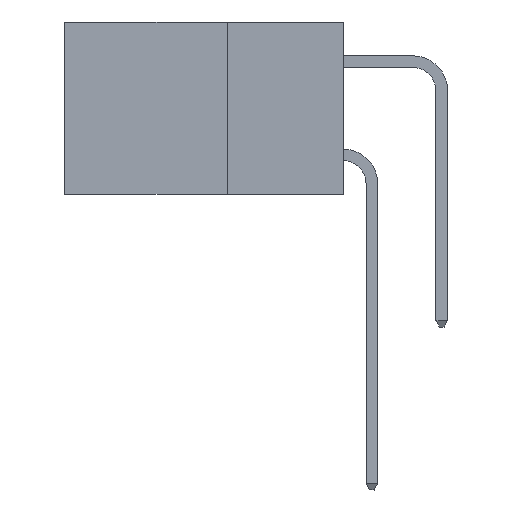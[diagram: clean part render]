
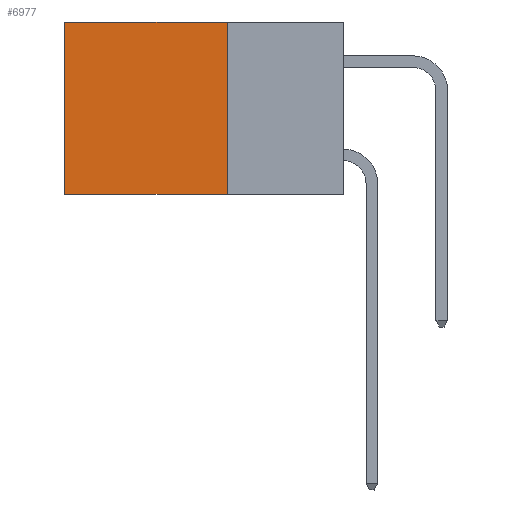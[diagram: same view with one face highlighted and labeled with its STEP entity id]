
A CAD part, left-side view. The second image highlights one B-rep face of the part: STEP entity #6977.
In plain terms, the highlighted planar face has unit normal (-1, 0, 0).
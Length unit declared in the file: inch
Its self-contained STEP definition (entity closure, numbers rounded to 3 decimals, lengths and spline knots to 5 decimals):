
#187 = CARTESIAN_POINT ( 'NONE',  ( 0.2615, 0.25, -0.37 ) ) ;
#285 = LINE ( 'NONE', #5379, #15265 ) ;
#374 = DIRECTION ( 'NONE',  ( 1., 0., 0. ) ) ;
#915 = CARTESIAN_POINT ( 'NONE',  ( 0.2615, 0.25, 0. ) ) ;
#1106 = ORIENTED_EDGE ( 'NONE', *, *, #14473, .T. ) ;
#1327 = DIRECTION ( 'NONE',  ( 0., 0., -1. ) ) ;
#1402 = ORIENTED_EDGE ( 'NONE', *, *, #2349, .F. ) ;
#2270 = VECTOR ( 'NONE', #15679, 39.37008 ) ;
#2349 = EDGE_CURVE ( 'NONE', #12914, #11816, #2787, .T. ) ;
#2787 = LINE ( 'NONE', #6552, #2270 ) ;
#3125 = DIRECTION ( 'NONE',  ( 0., 0., -1. ) ) ;
#4162 = VECTOR ( 'NONE', #15305, 39.37008 ) ;
#5379 = CARTESIAN_POINT ( 'NONE',  ( 0.2615, 0.25, -0.37 ) ) ;
#5733 = FACE_OUTER_BOUND ( 'NONE', #13371, .T. ) ;
#6552 = CARTESIAN_POINT ( 'NONE',  ( 0.2615, 0.25, -0.37 ) ) ;
#6977 = ADVANCED_FACE ( 'NONE', ( #5733 ), #13239, .F. ) ;
#7487 = LINE ( 'NONE', #14041, #11873 ) ;
#9412 = ORIENTED_EDGE ( 'NONE', *, *, #15561, .T. ) ;
#9952 = VERTEX_POINT ( 'NONE', #915 ) ;
#10226 = CARTESIAN_POINT ( 'NONE',  ( 0.2615, 0.25, 0. ) ) ;
#11066 = CARTESIAN_POINT ( 'NONE',  ( 0.2615, 0.6, 0. ) ) ;
#11247 = EDGE_CURVE ( 'NONE', #9952, #12914, #285, .T. ) ;
#11816 = VERTEX_POINT ( 'NONE', #15480 ) ;
#11873 = VECTOR ( 'NONE', #1327, 39.37008 ) ;
#11900 = CARTESIAN_POINT ( 'NONE',  ( 0.2615, 0.25, -0.37 ) ) ;
#12606 = AXIS2_PLACEMENT_3D ( 'NONE', #11900, #374, #3125 ) ;
#12862 = LINE ( 'NONE', #10226, #4162 ) ;
#12914 = VERTEX_POINT ( 'NONE', #187 ) ;
#13228 = DIRECTION ( 'NONE',  ( 0., 0., -1. ) ) ;
#13239 = PLANE ( 'NONE',  #12606 ) ;
#13371 = EDGE_LOOP ( 'NONE', ( #9412, #1402, #13930, #1106 ) ) ;
#13930 = ORIENTED_EDGE ( 'NONE', *, *, #11247, .F. ) ;
#14041 = CARTESIAN_POINT ( 'NONE',  ( 0.2615, 0.6, -0.37 ) ) ;
#14473 = EDGE_CURVE ( 'NONE', #9952, #16378, #12862, .T. ) ;
#15265 = VECTOR ( 'NONE', #13228, 39.37008 ) ;
#15305 = DIRECTION ( 'NONE',  ( 0., 1., 0. ) ) ;
#15480 = CARTESIAN_POINT ( 'NONE',  ( 0.2615, 0.6, -0.37 ) ) ;
#15561 = EDGE_CURVE ( 'NONE', #16378, #11816, #7487, .T. ) ;
#15679 = DIRECTION ( 'NONE',  ( 0., 1., 0. ) ) ;
#16378 = VERTEX_POINT ( 'NONE', #11066 ) ;
